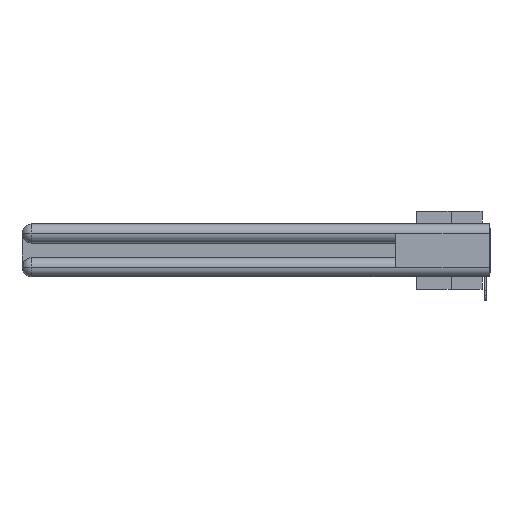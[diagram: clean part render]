
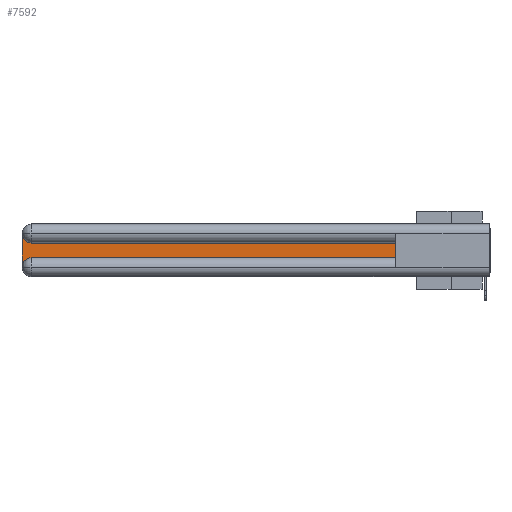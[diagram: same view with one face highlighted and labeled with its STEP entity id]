
A CAD part, left-side view. The second image highlights one B-rep face of the part: STEP entity #7592.
In plain terms, the highlighted planar face has unit normal (-1, 0, 0).
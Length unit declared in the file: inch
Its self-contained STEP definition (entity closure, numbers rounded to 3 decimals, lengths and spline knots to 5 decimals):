
#129 = VERTEX_POINT ( 'NONE', #26668 ) ;
#398 = DIRECTION ( 'NONE',  ( 0., 0., -1. ) ) ;
#947 = VECTOR ( 'NONE', #17781, 39.37008 ) ;
#2300 = CARTESIAN_POINT ( 'NONE',  ( 0.075, 0.6, -0.2175 ) ) ;
#3557 = ORIENTED_EDGE ( 'NONE', *, *, #9480, .T. ) ;
#3649 = EDGE_CURVE ( 'NONE', #21903, #129, #16568, .T. ) ;
#3942 = CARTESIAN_POINT ( 'NONE',  ( 0.075, 2.94, -0.2175 ) ) ;
#4290 = ORIENTED_EDGE ( 'NONE', *, *, #25224, .T. ) ;
#5015 = VERTEX_POINT ( 'NONE', #24468 ) ;
#7263 = AXIS2_PLACEMENT_3D ( 'NONE', #24203, #7969, #21888 ) ;
#7293 = FACE_OUTER_BOUND ( 'NONE', #25806, .T. ) ;
#7592 = ADVANCED_FACE ( 'NONE', ( #7293 ), #12425, .F. ) ;
#7969 = DIRECTION ( 'NONE',  ( 1., 0., 0. ) ) ;
#8207 = VERTEX_POINT ( 'NONE', #14538 ) ;
#8924 = ORIENTED_EDGE ( 'NONE', *, *, #3649, .T. ) ;
#9140 = EDGE_CURVE ( 'NONE', #13624, #21903, #14807, .T. ) ;
#9273 = CIRCLE ( 'NONE', #9723, 0.06 ) ;
#9462 = AXIS2_PLACEMENT_3D ( 'NONE', #10194, #26112, #12228 ) ;
#9480 = EDGE_CURVE ( 'NONE', #8207, #5015, #29295, .T. ) ;
#9723 = AXIS2_PLACEMENT_3D ( 'NONE', #10527, #10735, #17512 ) ;
#10194 = CARTESIAN_POINT ( 'NONE',  ( 0.075, 3., -0.1225 ) ) ;
#10527 = CARTESIAN_POINT ( 'NONE',  ( 0.075, 2.94, -0.2775 ) ) ;
#10735 = DIRECTION ( 'NONE',  ( 1., 0., 0. ) ) ;
#11914 = VECTOR ( 'NONE', #398, 39.37008 ) ;
#12228 = DIRECTION ( 'NONE',  ( 0., 0., -1. ) ) ;
#12425 = PLANE ( 'NONE',  #9462 ) ;
#13241 = DIRECTION ( 'NONE',  ( 0., -1., 0. ) ) ;
#13624 = VERTEX_POINT ( 'NONE', #3942 ) ;
#13977 = ORIENTED_EDGE ( 'NONE', *, *, #9140, .T. ) ;
#14193 = EDGE_CURVE ( 'NONE', #129, #27608, #18045, .T. ) ;
#14216 = CARTESIAN_POINT ( 'NONE',  ( 0.075, 0.6, -0.1225 ) ) ;
#14286 = ORIENTED_EDGE ( 'NONE', *, *, #14193, .T. ) ;
#14538 = CARTESIAN_POINT ( 'NONE',  ( 0.075, 3., -0.0625 ) ) ;
#14807 = LINE ( 'NONE', #22606, #19532 ) ;
#16568 = LINE ( 'NONE', #20028, #947 ) ;
#17512 = DIRECTION ( 'NONE',  ( 0., 0., -1. ) ) ;
#17781 = DIRECTION ( 'NONE',  ( 0., 0., 1. ) ) ;
#18045 = LINE ( 'NONE', #14216, #19465 ) ;
#19148 = CIRCLE ( 'NONE', #7263, 0.06 ) ;
#19465 = VECTOR ( 'NONE', #28007, 39.37008 ) ;
#19532 = VECTOR ( 'NONE', #13241, 39.37008 ) ;
#20028 = CARTESIAN_POINT ( 'NONE',  ( 0.075, 0.6, -0.2175 ) ) ;
#20786 = ORIENTED_EDGE ( 'NONE', *, *, #21222, .T. ) ;
#21116 = CARTESIAN_POINT ( 'NONE',  ( 0.075, 2.94, -0.1225 ) ) ;
#21222 = EDGE_CURVE ( 'NONE', #5015, #13624, #9273, .T. ) ;
#21888 = DIRECTION ( 'NONE',  ( 0., 0., -1. ) ) ;
#21903 = VERTEX_POINT ( 'NONE', #2300 ) ;
#22606 = CARTESIAN_POINT ( 'NONE',  ( 0.075, 0.6, -0.2175 ) ) ;
#24203 = CARTESIAN_POINT ( 'NONE',  ( 0.075, 2.94, -0.0625 ) ) ;
#24468 = CARTESIAN_POINT ( 'NONE',  ( 0.075, 3., -0.2775 ) ) ;
#25224 = EDGE_CURVE ( 'NONE', #27608, #8207, #19148, .T. ) ;
#25806 = EDGE_LOOP ( 'NONE', ( #14286, #4290, #3557, #20786, #13977, #8924 ) ) ;
#26112 = DIRECTION ( 'NONE',  ( 1., 0., 0. ) ) ;
#26668 = CARTESIAN_POINT ( 'NONE',  ( 0.075, 0.6, -0.1225 ) ) ;
#27608 = VERTEX_POINT ( 'NONE', #21116 ) ;
#28007 = DIRECTION ( 'NONE',  ( 0., 1., 0. ) ) ;
#28204 = CARTESIAN_POINT ( 'NONE',  ( 0.075, 3., -0.2175 ) ) ;
#29295 = LINE ( 'NONE', #28204, #11914 ) ;
